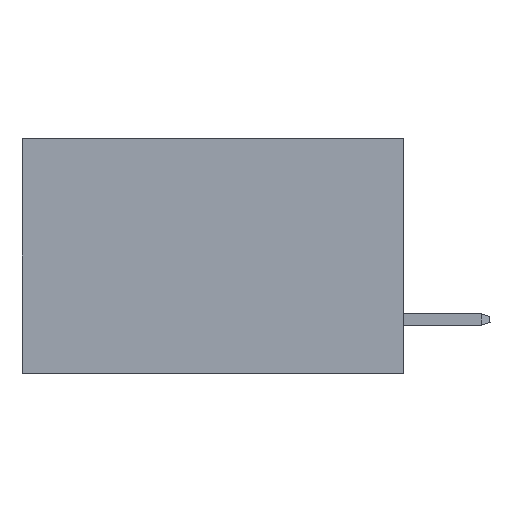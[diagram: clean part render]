
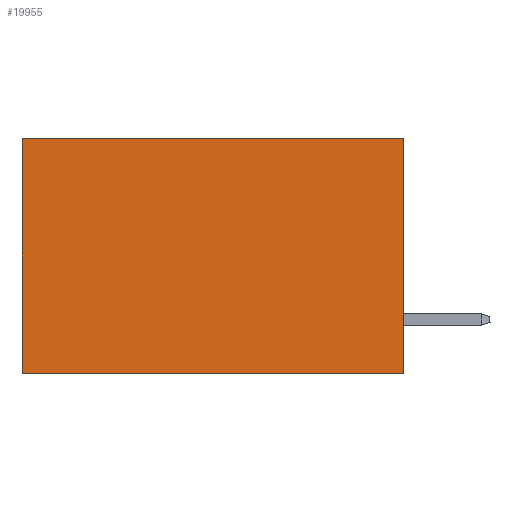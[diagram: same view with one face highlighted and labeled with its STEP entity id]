
A CAD part, left-side view. The second image highlights one B-rep face of the part: STEP entity #19955.
In plain terms, the highlighted planar face has unit normal (-1, 0, 0).
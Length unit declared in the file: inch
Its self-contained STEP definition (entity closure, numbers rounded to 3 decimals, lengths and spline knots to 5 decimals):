
#155 = CARTESIAN_POINT ( 'NONE',  ( 0.2875, 0., -0.37 ) ) ;
#504 = AXIS2_PLACEMENT_3D ( 'NONE', #5920, #2527, #18450 ) ;
#1088 = CARTESIAN_POINT ( 'NONE',  ( 0.2875, 0.6, 0. ) ) ;
#2086 = ORIENTED_EDGE ( 'NONE', *, *, #10214, .F. ) ;
#2150 = VERTEX_POINT ( 'NONE', #1088 ) ;
#2527 = DIRECTION ( 'NONE',  ( 1., 0., 0. ) ) ;
#2840 = CARTESIAN_POINT ( 'NONE',  ( 0.2875, 0.6, -0.37 ) ) ;
#2914 = CARTESIAN_POINT ( 'NONE',  ( 0.2875, 0.6, 0. ) ) ;
#3476 = CARTESIAN_POINT ( 'NONE',  ( 0.2875, 0., 0. ) ) ;
#4424 = DIRECTION ( 'NONE',  ( 0., 1., 0. ) ) ;
#5302 = EDGE_CURVE ( 'NONE', #13330, #11435, #18241, .T. ) ;
#5920 = CARTESIAN_POINT ( 'NONE',  ( 0.2875, 0., 0. ) ) ;
#6099 = DIRECTION ( 'NONE',  ( 0., 0., -1. ) ) ;
#6110 = VECTOR ( 'NONE', #15374, 39.37008 ) ;
#6863 = EDGE_CURVE ( 'NONE', #2150, #15393, #17716, .T. ) ;
#9287 = VECTOR ( 'NONE', #9880, 39.37008 ) ;
#9793 = ORIENTED_EDGE ( 'NONE', *, *, #6863, .T. ) ;
#9880 = DIRECTION ( 'NONE',  ( 0., 1., 0. ) ) ;
#10214 = EDGE_CURVE ( 'NONE', #11435, #15393, #17466, .T. ) ;
#10648 = CARTESIAN_POINT ( 'NONE',  ( 0.2875, 0., 0. ) ) ;
#11314 = EDGE_LOOP ( 'NONE', ( #9793, #2086, #18337, #12703 ) ) ;
#11410 = VECTOR ( 'NONE', #6099, 39.37008 ) ;
#11435 = VERTEX_POINT ( 'NONE', #155 ) ;
#12285 = FACE_OUTER_BOUND ( 'NONE', #11314, .T. ) ;
#12703 = ORIENTED_EDGE ( 'NONE', *, *, #19694, .T. ) ;
#13330 = VERTEX_POINT ( 'NONE', #15727 ) ;
#13786 = LINE ( 'NONE', #3476, #18855 ) ;
#15374 = DIRECTION ( 'NONE',  ( 0., 0., -1. ) ) ;
#15393 = VERTEX_POINT ( 'NONE', #2840 ) ;
#15727 = CARTESIAN_POINT ( 'NONE',  ( 0.2875, 0., 0. ) ) ;
#16613 = PLANE ( 'NONE',  #504 ) ;
#17466 = LINE ( 'NONE', #17765, #9287 ) ;
#17716 = LINE ( 'NONE', #2914, #11410 ) ;
#17765 = CARTESIAN_POINT ( 'NONE',  ( 0.2875, 0., -0.37 ) ) ;
#18241 = LINE ( 'NONE', #10648, #6110 ) ;
#18337 = ORIENTED_EDGE ( 'NONE', *, *, #5302, .F. ) ;
#18450 = DIRECTION ( 'NONE',  ( 0., 0., -1. ) ) ;
#18855 = VECTOR ( 'NONE', #4424, 39.37008 ) ;
#19694 = EDGE_CURVE ( 'NONE', #13330, #2150, #13786, .T. ) ;
#19955 = ADVANCED_FACE ( 'NONE', ( #12285 ), #16613, .F. ) ;
